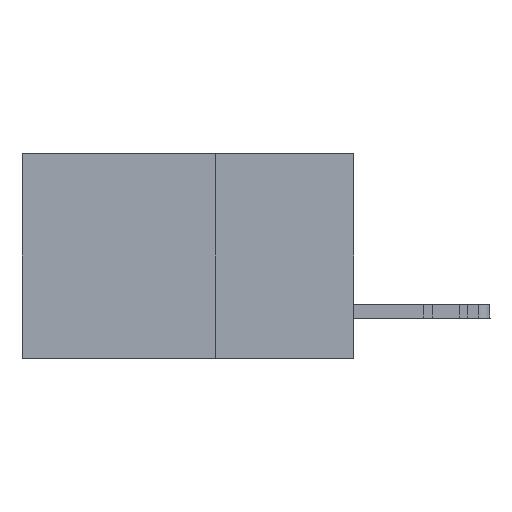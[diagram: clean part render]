
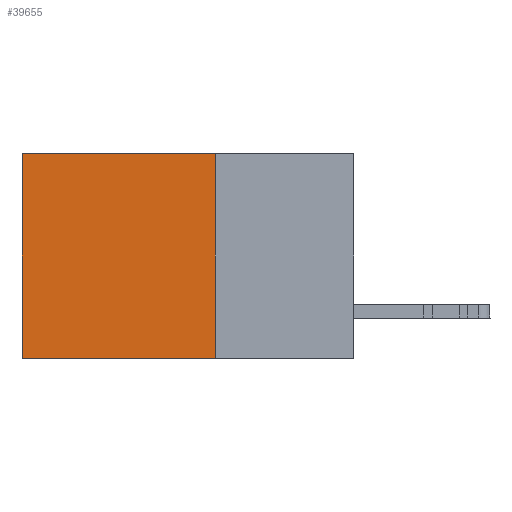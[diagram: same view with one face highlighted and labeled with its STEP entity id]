
A CAD part, left-side view. The second image highlights one B-rep face of the part: STEP entity #39655.
In plain terms, the highlighted planar face has unit normal (-1, 0, 0).
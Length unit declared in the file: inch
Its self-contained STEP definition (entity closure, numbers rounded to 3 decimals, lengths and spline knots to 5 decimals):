
#614 = VERTEX_POINT ( 'NONE', #48248 ) ;
#1561 = CARTESIAN_POINT ( 'NONE',  ( 0.2875, 0.6, 0. ) ) ;
#2166 = LINE ( 'NONE', #7839, #4077 ) ;
#4077 = VECTOR ( 'NONE', #43465, 39.37008 ) ;
#4739 = FACE_OUTER_BOUND ( 'NONE', #14665, .T. ) ;
#6041 = AXIS2_PLACEMENT_3D ( 'NONE', #46894, #11382, #27399 ) ;
#6309 = ORIENTED_EDGE ( 'NONE', *, *, #14701, .T. ) ;
#7839 = CARTESIAN_POINT ( 'NONE',  ( 0.2875, 0.25, 0. ) ) ;
#11382 = DIRECTION ( 'NONE',  ( 1., 0., 0. ) ) ;
#11637 = ORIENTED_EDGE ( 'NONE', *, *, #41942, .F. ) ;
#14483 = VERTEX_POINT ( 'NONE', #44871 ) ;
#14665 = EDGE_LOOP ( 'NONE', ( #6309, #21840, #11637, #36331 ) ) ;
#14701 = EDGE_CURVE ( 'NONE', #25667, #614, #15942, .T. ) ;
#15942 = LINE ( 'NONE', #1561, #23897 ) ;
#17765 = CARTESIAN_POINT ( 'NONE',  ( 0.2875, 0.25, 0. ) ) ;
#21840 = ORIENTED_EDGE ( 'NONE', *, *, #37242, .F. ) ;
#22187 = VECTOR ( 'NONE', #40313, 39.37008 ) ;
#23897 = VECTOR ( 'NONE', #33114, 39.37008 ) ;
#24248 = PLANE ( 'NONE',  #6041 ) ;
#25667 = VERTEX_POINT ( 'NONE', #44983 ) ;
#26443 = LINE ( 'NONE', #17765, #44639 ) ;
#27399 = DIRECTION ( 'NONE',  ( 0., 0., -1. ) ) ;
#28471 = CARTESIAN_POINT ( 'NONE',  ( 0.2875, 0.25, -0.37 ) ) ;
#33114 = DIRECTION ( 'NONE',  ( 0., 0., -1. ) ) ;
#34561 = CARTESIAN_POINT ( 'NONE',  ( 0.2875, 0.25, -0.37 ) ) ;
#36211 = LINE ( 'NONE', #28471, #22187 ) ;
#36331 = ORIENTED_EDGE ( 'NONE', *, *, #40931, .T. ) ;
#37242 = EDGE_CURVE ( 'NONE', #37330, #614, #36211, .T. ) ;
#37330 = VERTEX_POINT ( 'NONE', #34561 ) ;
#37659 = DIRECTION ( 'NONE',  ( 0., 0., -1. ) ) ;
#39655 = ADVANCED_FACE ( 'NONE', ( #4739 ), #24248, .F. ) ;
#40313 = DIRECTION ( 'NONE',  ( 0., 1., 0. ) ) ;
#40931 = EDGE_CURVE ( 'NONE', #14483, #25667, #2166, .T. ) ;
#41942 = EDGE_CURVE ( 'NONE', #14483, #37330, #26443, .T. ) ;
#43465 = DIRECTION ( 'NONE',  ( 0., 1., 0. ) ) ;
#44639 = VECTOR ( 'NONE', #37659, 39.37008 ) ;
#44871 = CARTESIAN_POINT ( 'NONE',  ( 0.2875, 0.25, 0. ) ) ;
#44983 = CARTESIAN_POINT ( 'NONE',  ( 0.2875, 0.6, 0. ) ) ;
#46894 = CARTESIAN_POINT ( 'NONE',  ( 0.2875, 0.25, 0. ) ) ;
#48248 = CARTESIAN_POINT ( 'NONE',  ( 0.2875, 0.6, -0.37 ) ) ;
